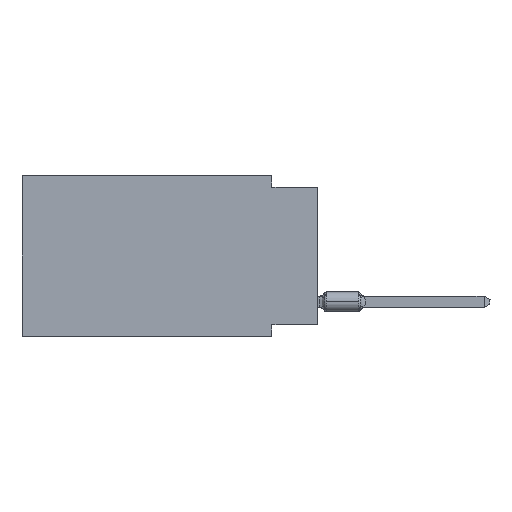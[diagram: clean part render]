
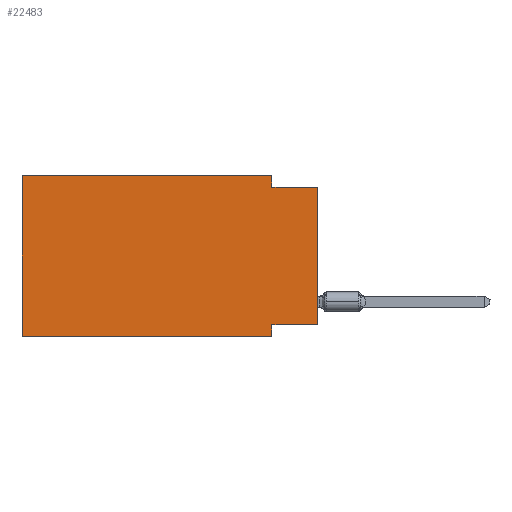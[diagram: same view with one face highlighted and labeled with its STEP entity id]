
A CAD part, left-side view. The second image highlights one B-rep face of the part: STEP entity #22483.
In plain terms, the highlighted planar face has unit normal (-1, 0, 0).
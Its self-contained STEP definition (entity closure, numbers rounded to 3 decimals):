
#1020 = VERTEX_POINT ( 'NONE', #30621 ) ;
#1170 = VERTEX_POINT ( 'NONE', #13936 ) ;
#1606 = LINE ( 'NONE', #55685, #44565 ) ;
#2573 = ORIENTED_EDGE ( 'NONE', *, *, #44297, .T. ) ;
#2664 = AXIS2_PLACEMENT_3D ( 'NONE', #45400, #8576, #35920 ) ;
#5415 = VECTOR ( 'NONE', #7045, 1000. ) ;
#7045 = DIRECTION ( 'NONE',  ( 0., -1., 0. ) ) ;
#8576 = DIRECTION ( 'NONE',  ( 1., 0., 0. ) ) ;
#8821 = DIRECTION ( 'NONE',  ( 0., 0., 1. ) ) ;
#8851 = PLANE ( 'NONE',  #2664 ) ;
#9767 = VERTEX_POINT ( 'NONE', #11286 ) ;
#9879 = VERTEX_POINT ( 'NONE', #43970 ) ;
#10426 = LINE ( 'NONE', #55301, #57340 ) ;
#10656 = EDGE_LOOP ( 'NONE', ( #50944, #16531, #29242, #13508, #48258, #2573, #52748, #23401 ) ) ;
#11286 = CARTESIAN_POINT ( 'NONE',  ( 0., 0., -8.255 ) ) ;
#12717 = FACE_OUTER_BOUND ( 'NONE', #10656, .T. ) ;
#13508 = ORIENTED_EDGE ( 'NONE', *, *, #49406, .F. ) ;
#13624 = DIRECTION ( 'NONE',  ( 0., -1., 0. ) ) ;
#13936 = CARTESIAN_POINT ( 'NONE',  ( 0., 16.383, -8.89 ) ) ;
#16531 = ORIENTED_EDGE ( 'NONE', *, *, #46481, .F. ) ;
#19514 = CARTESIAN_POINT ( 'NONE',  ( 0., 2.54, -8.89 ) ) ;
#19908 = VERTEX_POINT ( 'NONE', #38488 ) ;
#20748 = CARTESIAN_POINT ( 'NONE',  ( 0., 0., -0.635 ) ) ;
#22483 = ADVANCED_FACE ( 'NONE', ( #12717 ), #8851, .F. ) ;
#23401 = ORIENTED_EDGE ( 'NONE', *, *, #53093, .F. ) ;
#23916 = DIRECTION ( 'NONE',  ( 0., -1., 0. ) ) ;
#24712 = DIRECTION ( 'NONE',  ( 0., 0., -1. ) ) ;
#26067 = LINE ( 'NONE', #34404, #56674 ) ;
#28040 = VECTOR ( 'NONE', #23916, 1000. ) ;
#29242 = ORIENTED_EDGE ( 'NONE', *, *, #32520, .F. ) ;
#30621 = CARTESIAN_POINT ( 'NONE',  ( 0., 2.54, -0.635 ) ) ;
#31256 = VECTOR ( 'NONE', #24712, 1000. ) ;
#32332 = CARTESIAN_POINT ( 'NONE',  ( 0., 16.383, 0. ) ) ;
#32520 = EDGE_CURVE ( 'NONE', #19908, #1020, #1606, .T. ) ;
#34404 = CARTESIAN_POINT ( 'NONE',  ( 0., 0., -8.255 ) ) ;
#35366 = LINE ( 'NONE', #40114, #55414 ) ;
#35920 = DIRECTION ( 'NONE',  ( 0., 0., -1. ) ) ;
#36035 = LINE ( 'NONE', #54148, #31256 ) ;
#38488 = CARTESIAN_POINT ( 'NONE',  ( 0., 2.54, 0. ) ) ;
#38800 = EDGE_CURVE ( 'NONE', #57888, #52477, #36035, .T. ) ;
#39153 = DIRECTION ( 'NONE',  ( 0., 1., 0. ) ) ;
#39762 = CARTESIAN_POINT ( 'NONE',  ( 0., 0., 0. ) ) ;
#40114 = CARTESIAN_POINT ( 'NONE',  ( 0., 16.383, 0. ) ) ;
#41434 = CARTESIAN_POINT ( 'NONE',  ( 0., 16.383, -8.89 ) ) ;
#41596 = CARTESIAN_POINT ( 'NONE',  ( 0., 2.54, -8.255 ) ) ;
#42330 = DIRECTION ( 'NONE',  ( 0., 0., -1. ) ) ;
#42632 = LINE ( 'NONE', #41434, #28040 ) ;
#43308 = LINE ( 'NONE', #20748, #5415 ) ;
#43502 = EDGE_CURVE ( 'NONE', #1170, #58179, #10426, .T. ) ;
#43970 = CARTESIAN_POINT ( 'NONE',  ( 0., 0., -0.635 ) ) ;
#44297 = EDGE_CURVE ( 'NONE', #1170, #52477, #42632, .T. ) ;
#44565 = VECTOR ( 'NONE', #42330, 1000. ) ;
#45400 = CARTESIAN_POINT ( 'NONE',  ( 0., 16.383, 0. ) ) ;
#45809 = DIRECTION ( 'NONE',  ( 0., 0., 1. ) ) ;
#46481 = EDGE_CURVE ( 'NONE', #1020, #9879, #43308, .T. ) ;
#48258 = ORIENTED_EDGE ( 'NONE', *, *, #43502, .F. ) ;
#48952 = LINE ( 'NONE', #39762, #55547 ) ;
#49406 = EDGE_CURVE ( 'NONE', #58179, #19908, #35366, .T. ) ;
#50944 = ORIENTED_EDGE ( 'NONE', *, *, #50961, .T. ) ;
#50961 = EDGE_CURVE ( 'NONE', #9767, #9879, #48952, .T. ) ;
#52477 = VERTEX_POINT ( 'NONE', #19514 ) ;
#52748 = ORIENTED_EDGE ( 'NONE', *, *, #38800, .F. ) ;
#53093 = EDGE_CURVE ( 'NONE', #9767, #57888, #26067, .T. ) ;
#54148 = CARTESIAN_POINT ( 'NONE',  ( 0., 2.54, -8.89 ) ) ;
#55301 = CARTESIAN_POINT ( 'NONE',  ( 0., 16.383, 0. ) ) ;
#55414 = VECTOR ( 'NONE', #13624, 1000. ) ;
#55547 = VECTOR ( 'NONE', #8821, 1000. ) ;
#55685 = CARTESIAN_POINT ( 'NONE',  ( 0., 2.54, 0. ) ) ;
#56674 = VECTOR ( 'NONE', #39153, 1000. ) ;
#57340 = VECTOR ( 'NONE', #45809, 1000. ) ;
#57888 = VERTEX_POINT ( 'NONE', #41596 ) ;
#58179 = VERTEX_POINT ( 'NONE', #32332 ) ;
